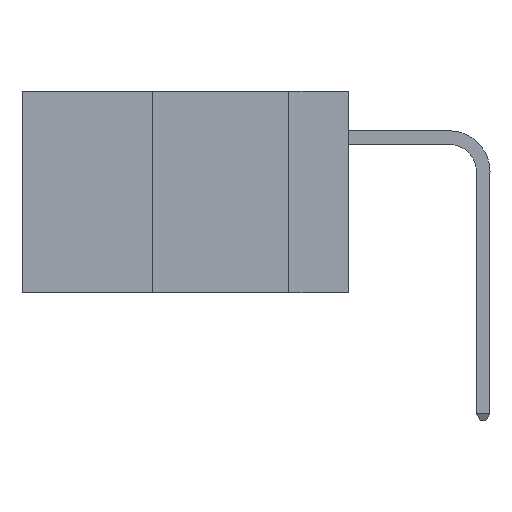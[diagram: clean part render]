
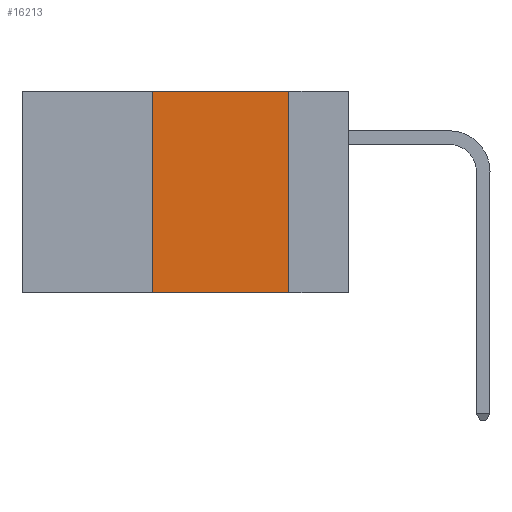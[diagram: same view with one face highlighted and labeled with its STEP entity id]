
A CAD part, left-side view. The second image highlights one B-rep face of the part: STEP entity #16213.
In plain terms, the highlighted planar face has unit normal (-1, 0, 0).
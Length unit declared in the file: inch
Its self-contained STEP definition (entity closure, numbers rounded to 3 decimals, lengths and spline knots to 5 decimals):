
#128 = VECTOR ( 'NONE', #10147, 39.37008 ) ;
#745 = CARTESIAN_POINT ( 'NONE',  ( 0., 0.6, 0. ) ) ;
#1963 = AXIS2_PLACEMENT_3D ( 'NONE', #745, #4009, #2423 ) ;
#1982 = VECTOR ( 'NONE', #11930, 39.37008 ) ;
#2017 = VECTOR ( 'NONE', #4375, 39.37008 ) ;
#2209 = EDGE_CURVE ( 'NONE', #3239, #19025, #5855, .T. ) ;
#2423 = DIRECTION ( 'NONE',  ( 0., 0., -1. ) ) ;
#3239 = VERTEX_POINT ( 'NONE', #19625 ) ;
#4009 = DIRECTION ( 'NONE',  ( 1., 0., 0. ) ) ;
#4275 = EDGE_CURVE ( 'NONE', #9437, #13397, #8937, .T. ) ;
#4375 = DIRECTION ( 'NONE',  ( 0., -1., 0. ) ) ;
#5121 = CARTESIAN_POINT ( 'NONE',  ( 0., 0.11, -0.37 ) ) ;
#5301 = CARTESIAN_POINT ( 'NONE',  ( 0., 0.36, 0. ) ) ;
#5855 = LINE ( 'NONE', #10081, #2017 ) ;
#6050 = CARTESIAN_POINT ( 'NONE',  ( 0., 0.6, 0. ) ) ;
#6087 = CARTESIAN_POINT ( 'NONE',  ( 0., 0.11, 0. ) ) ;
#7289 = DIRECTION ( 'NONE',  ( 0., -1., 0. ) ) ;
#7785 = ORIENTED_EDGE ( 'NONE', *, *, #18256, .F. ) ;
#8937 = LINE ( 'NONE', #6050, #20505 ) ;
#9437 = VERTEX_POINT ( 'NONE', #5301 ) ;
#10081 = CARTESIAN_POINT ( 'NONE',  ( 0., 0.6, -0.37 ) ) ;
#10147 = DIRECTION ( 'NONE',  ( 0., 0., -1. ) ) ;
#10297 = FACE_OUTER_BOUND ( 'NONE', #16798, .T. ) ;
#11930 = DIRECTION ( 'NONE',  ( 0., 0., 1. ) ) ;
#13397 = VERTEX_POINT ( 'NONE', #6087 ) ;
#13681 = EDGE_CURVE ( 'NONE', #3239, #9437, #18240, .T. ) ;
#13735 = PLANE ( 'NONE',  #1963 ) ;
#14010 = ORIENTED_EDGE ( 'NONE', *, *, #13681, .F. ) ;
#16213 = ADVANCED_FACE ( 'NONE', ( #10297 ), #13735, .F. ) ;
#16798 = EDGE_LOOP ( 'NONE', ( #7785, #18381, #14010, #21225 ) ) ;
#18240 = LINE ( 'NONE', #19786, #1982 ) ;
#18256 = EDGE_CURVE ( 'NONE', #13397, #19025, #18715, .T. ) ;
#18381 = ORIENTED_EDGE ( 'NONE', *, *, #4275, .F. ) ;
#18382 = CARTESIAN_POINT ( 'NONE',  ( 0., 0.11, 0. ) ) ;
#18715 = LINE ( 'NONE', #18382, #128 ) ;
#19025 = VERTEX_POINT ( 'NONE', #5121 ) ;
#19625 = CARTESIAN_POINT ( 'NONE',  ( 0., 0.36, -0.37 ) ) ;
#19786 = CARTESIAN_POINT ( 'NONE',  ( 0., 0.36, 0. ) ) ;
#20505 = VECTOR ( 'NONE', #7289, 39.37008 ) ;
#21225 = ORIENTED_EDGE ( 'NONE', *, *, #2209, .T. ) ;
